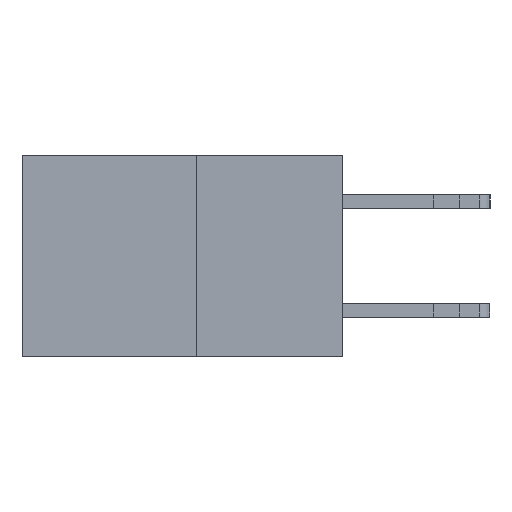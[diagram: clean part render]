
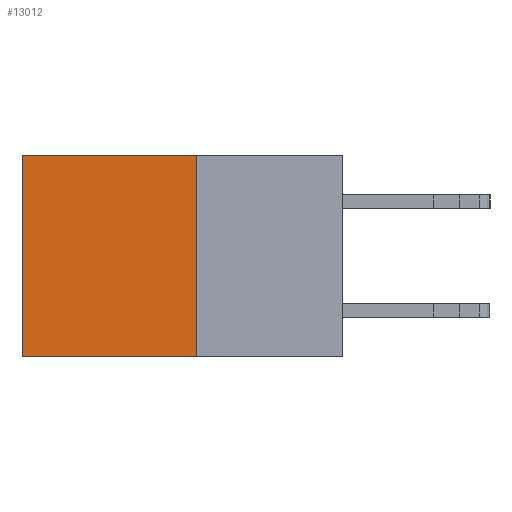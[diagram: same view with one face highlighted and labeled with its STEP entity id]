
A CAD part, left-side view. The second image highlights one B-rep face of the part: STEP entity #13012.
In plain terms, the highlighted planar face has unit normal (-1, 0, 0).
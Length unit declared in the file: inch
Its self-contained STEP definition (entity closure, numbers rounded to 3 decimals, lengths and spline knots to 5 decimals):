
#270 = PLANE ( 'NONE',  #1174 ) ;
#413 = DIRECTION ( 'NONE',  ( 0., 1., 0. ) ) ;
#662 = CARTESIAN_POINT ( 'NONE',  ( 0.277, 0.59, 0. ) ) ;
#1098 = ORIENTED_EDGE ( 'NONE', *, *, #12829, .F. ) ;
#1174 = AXIS2_PLACEMENT_3D ( 'NONE', #8481, #1432, #9667 ) ;
#1432 = DIRECTION ( 'NONE',  ( 1., 0., 0. ) ) ;
#1782 = DIRECTION ( 'NONE',  ( 0., 0., -1. ) ) ;
#1803 = CARTESIAN_POINT ( 'NONE',  ( 0.277, 0.27, -0.37 ) ) ;
#3125 = EDGE_CURVE ( 'NONE', #6351, #11655, #8833, .T. ) ;
#3215 = ORIENTED_EDGE ( 'NONE', *, *, #9820, .T. ) ;
#3280 = LINE ( 'NONE', #1803, #12311 ) ;
#3392 = CARTESIAN_POINT ( 'NONE',  ( 0.277, 0.27, -0.37 ) ) ;
#3543 = EDGE_CURVE ( 'NONE', #11308, #7618, #3280, .T. ) ;
#4130 = FACE_OUTER_BOUND ( 'NONE', #11587, .T. ) ;
#4586 = DIRECTION ( 'NONE',  ( 0., 1., 0. ) ) ;
#5911 = CARTESIAN_POINT ( 'NONE',  ( 0.277, 0.27, -0.37 ) ) ;
#6351 = VERTEX_POINT ( 'NONE', #662 ) ;
#6699 = LINE ( 'NONE', #3392, #10219 ) ;
#7618 = VERTEX_POINT ( 'NONE', #5911 ) ;
#7737 = LINE ( 'NONE', #12118, #10500 ) ;
#8481 = CARTESIAN_POINT ( 'NONE',  ( 0.277, 0.27, -0.37 ) ) ;
#8833 = LINE ( 'NONE', #9695, #14691 ) ;
#9266 = DIRECTION ( 'NONE',  ( 0., 0., -1. ) ) ;
#9616 = CARTESIAN_POINT ( 'NONE',  ( 0.277, 0.59, -0.37 ) ) ;
#9667 = DIRECTION ( 'NONE',  ( 0., 0., -1. ) ) ;
#9695 = CARTESIAN_POINT ( 'NONE',  ( 0.277, 0.59, -0.37 ) ) ;
#9820 = EDGE_CURVE ( 'NONE', #11308, #6351, #7737, .T. ) ;
#10142 = CARTESIAN_POINT ( 'NONE',  ( 0.277, 0.27, 0. ) ) ;
#10219 = VECTOR ( 'NONE', #4586, 39.37008 ) ;
#10500 = VECTOR ( 'NONE', #413, 39.37008 ) ;
#11308 = VERTEX_POINT ( 'NONE', #10142 ) ;
#11587 = EDGE_LOOP ( 'NONE', ( #11790, #1098, #14137, #3215 ) ) ;
#11655 = VERTEX_POINT ( 'NONE', #9616 ) ;
#11790 = ORIENTED_EDGE ( 'NONE', *, *, #3125, .T. ) ;
#12118 = CARTESIAN_POINT ( 'NONE',  ( 0.277, 0.27, 0. ) ) ;
#12311 = VECTOR ( 'NONE', #1782, 39.37008 ) ;
#12829 = EDGE_CURVE ( 'NONE', #7618, #11655, #6699, .T. ) ;
#13012 = ADVANCED_FACE ( 'NONE', ( #4130 ), #270, .F. ) ;
#14137 = ORIENTED_EDGE ( 'NONE', *, *, #3543, .F. ) ;
#14691 = VECTOR ( 'NONE', #9266, 39.37008 ) ;
